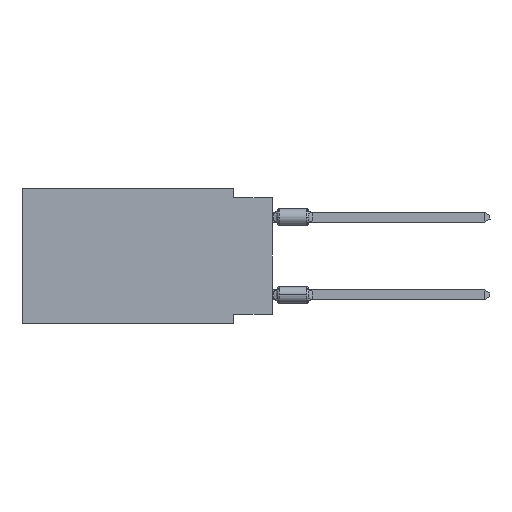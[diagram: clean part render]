
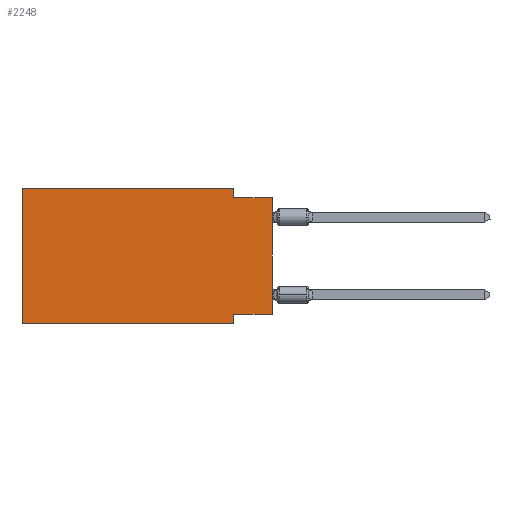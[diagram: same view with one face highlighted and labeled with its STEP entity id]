
A CAD part, left-side view. The second image highlights one B-rep face of the part: STEP entity #2248.
In plain terms, the highlighted planar face has unit normal (-1, 0, 0).
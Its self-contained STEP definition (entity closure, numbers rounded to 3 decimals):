
#1725 = VECTOR ( 'NONE', #46956, 1000. ) ;
#1733 = VECTOR ( 'NONE', #41345, 1000. ) ;
#2248 = ADVANCED_FACE ( 'NONE', ( #58908 ), #42134, .F. ) ;
#2523 = VECTOR ( 'NONE', #20085, 1000. ) ;
#2535 = VERTEX_POINT ( 'NONE', #34432 ) ;
#3173 = LINE ( 'NONE', #69541, #34252 ) ;
#3532 = CARTESIAN_POINT ( 'NONE',  ( 0., 16.383, -8.89 ) ) ;
#3783 = CARTESIAN_POINT ( 'NONE',  ( 0., 0., -8.255 ) ) ;
#6160 = ORIENTED_EDGE ( 'NONE', *, *, #9965, .F. ) ;
#7254 = VECTOR ( 'NONE', #18749, 1000. ) ;
#8305 = LINE ( 'NONE', #36032, #68196 ) ;
#8836 = CARTESIAN_POINT ( 'NONE',  ( 0., 0., -8.255 ) ) ;
#8942 = DIRECTION ( 'NONE',  ( 1., 0., 0. ) ) ;
#9965 = EDGE_CURVE ( 'NONE', #23353, #22240, #20055, .T. ) ;
#12694 = CARTESIAN_POINT ( 'NONE',  ( 0., 2.54, 0. ) ) ;
#12805 = EDGE_CURVE ( 'NONE', #34542, #27802, #25615, .T. ) ;
#13774 = CARTESIAN_POINT ( 'NONE',  ( 0., 16.383, 0. ) ) ;
#13955 = EDGE_CURVE ( 'NONE', #44249, #23353, #30908, .T. ) ;
#14714 = LINE ( 'NONE', #30405, #7254 ) ;
#14782 = CARTESIAN_POINT ( 'NONE',  ( 0., 16.383, 0. ) ) ;
#16032 = ORIENTED_EDGE ( 'NONE', *, *, #51170, .T. ) ;
#16237 = EDGE_CURVE ( 'NONE', #27802, #49802, #8305, .T. ) ;
#18749 = DIRECTION ( 'NONE',  ( 0., -1., 0. ) ) ;
#19224 = CARTESIAN_POINT ( 'NONE',  ( 0., 2.54, -0.635 ) ) ;
#20055 = LINE ( 'NONE', #52528, #29144 ) ;
#20085 = DIRECTION ( 'NONE',  ( 0., 0., 1. ) ) ;
#21876 = DIRECTION ( 'NONE',  ( 0., 1., 0. ) ) ;
#22240 = VERTEX_POINT ( 'NONE', #19224 ) ;
#23353 = VERTEX_POINT ( 'NONE', #12694 ) ;
#23572 = ORIENTED_EDGE ( 'NONE', *, *, #12805, .F. ) ;
#25615 = LINE ( 'NONE', #8836, #29581 ) ;
#25889 = DIRECTION ( 'NONE',  ( 0., 0., -1. ) ) ;
#27480 = VERTEX_POINT ( 'NONE', #3532 ) ;
#27802 = VERTEX_POINT ( 'NONE', #30067 ) ;
#27969 = AXIS2_PLACEMENT_3D ( 'NONE', #14782, #8942, #46878 ) ;
#29144 = VECTOR ( 'NONE', #25889, 1000. ) ;
#29581 = VECTOR ( 'NONE', #21876, 1000. ) ;
#30067 = CARTESIAN_POINT ( 'NONE',  ( 0., 2.54, -8.255 ) ) ;
#30405 = CARTESIAN_POINT ( 'NONE',  ( 0., 0., -0.635 ) ) ;
#30549 = EDGE_LOOP ( 'NONE', ( #62986, #33882, #6160, #31435, #46533, #16032, #45881, #23572 ) ) ;
#30908 = LINE ( 'NONE', #13774, #1725 ) ;
#31435 = ORIENTED_EDGE ( 'NONE', *, *, #13955, .F. ) ;
#33882 = ORIENTED_EDGE ( 'NONE', *, *, #63362, .F. ) ;
#34252 = VECTOR ( 'NONE', #47647, 1000. ) ;
#34432 = CARTESIAN_POINT ( 'NONE',  ( 0., 0., -0.635 ) ) ;
#34542 = VERTEX_POINT ( 'NONE', #3783 ) ;
#35163 = LINE ( 'NONE', #57769, #1733 ) ;
#36032 = CARTESIAN_POINT ( 'NONE',  ( 0., 2.54, -8.89 ) ) ;
#41345 = DIRECTION ( 'NONE',  ( 0., 0., 1. ) ) ;
#42134 = PLANE ( 'NONE',  #27969 ) ;
#42166 = CARTESIAN_POINT ( 'NONE',  ( 0., 2.54, -8.89 ) ) ;
#44249 = VERTEX_POINT ( 'NONE', #51134 ) ;
#45881 = ORIENTED_EDGE ( 'NONE', *, *, #16237, .F. ) ;
#46533 = ORIENTED_EDGE ( 'NONE', *, *, #58151, .F. ) ;
#46878 = DIRECTION ( 'NONE',  ( 0., 0., -1. ) ) ;
#46956 = DIRECTION ( 'NONE',  ( 0., -1., 0. ) ) ;
#46961 = DIRECTION ( 'NONE',  ( 0., 0., -1. ) ) ;
#47647 = DIRECTION ( 'NONE',  ( 0., -1., 0. ) ) ;
#49802 = VERTEX_POINT ( 'NONE', #42166 ) ;
#51134 = CARTESIAN_POINT ( 'NONE',  ( 0., 16.383, 0. ) ) ;
#51170 = EDGE_CURVE ( 'NONE', #27480, #49802, #3173, .T. ) ;
#52528 = CARTESIAN_POINT ( 'NONE',  ( 0., 2.54, 0. ) ) ;
#53644 = LINE ( 'NONE', #70393, #2523 ) ;
#57769 = CARTESIAN_POINT ( 'NONE',  ( 0., 16.383, 0. ) ) ;
#58151 = EDGE_CURVE ( 'NONE', #27480, #44249, #35163, .T. ) ;
#58908 = FACE_OUTER_BOUND ( 'NONE', #30549, .T. ) ;
#62600 = EDGE_CURVE ( 'NONE', #34542, #2535, #53644, .T. ) ;
#62986 = ORIENTED_EDGE ( 'NONE', *, *, #62600, .T. ) ;
#63362 = EDGE_CURVE ( 'NONE', #22240, #2535, #14714, .T. ) ;
#68196 = VECTOR ( 'NONE', #46961, 1000. ) ;
#69541 = CARTESIAN_POINT ( 'NONE',  ( 0., 16.383, -8.89 ) ) ;
#70393 = CARTESIAN_POINT ( 'NONE',  ( 0., 0., 0. ) ) ;
